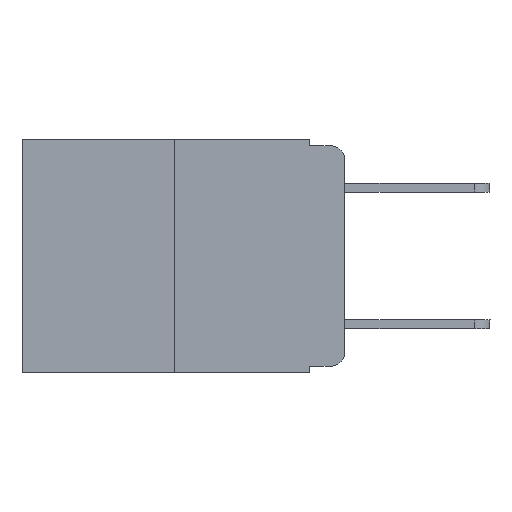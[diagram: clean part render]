
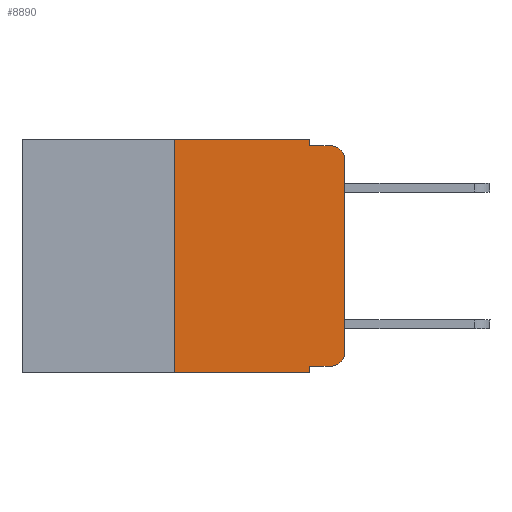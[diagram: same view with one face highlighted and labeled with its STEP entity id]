
A CAD part, left-side view. The second image highlights one B-rep face of the part: STEP entity #8890.
In plain terms, the highlighted planar face has unit normal (-1, 0, 0).
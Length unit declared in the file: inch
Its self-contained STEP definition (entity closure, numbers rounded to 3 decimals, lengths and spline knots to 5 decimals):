
#1074 = VERTEX_POINT ( 'NONE', #18819 ) ;
#1126 = VERTEX_POINT ( 'NONE', #11155 ) ;
#1210 = ORIENTED_EDGE ( 'NONE', *, *, #6990, .T. ) ;
#1225 = ORIENTED_EDGE ( 'NONE', *, *, #2847, .F. ) ;
#1250 = AXIS2_PLACEMENT_3D ( 'NONE', #14563, #1403, #7265 ) ;
#1403 = DIRECTION ( 'NONE',  ( -1., 0., 0. ) ) ;
#1538 = DIRECTION ( 'NONE',  ( 0., 0., -1. ) ) ;
#1814 = VERTEX_POINT ( 'NONE', #7582 ) ;
#2265 = DIRECTION ( 'NONE',  ( 0., 0., 1. ) ) ;
#2280 = VECTOR ( 'NONE', #1538, 39.37008 ) ;
#2627 = VERTEX_POINT ( 'NONE', #10776 ) ;
#2756 = DIRECTION ( 'NONE',  ( 0., 0., 1. ) ) ;
#2758 = CIRCLE ( 'NONE', #11976, 0.02 ) ;
#2847 = EDGE_CURVE ( 'NONE', #8914, #1814, #14785, .T. ) ;
#3296 = VECTOR ( 'NONE', #14700, 39.37008 ) ;
#3506 = EDGE_CURVE ( 'NONE', #2627, #1074, #11932, .T. ) ;
#3644 = ORIENTED_EDGE ( 'NONE', *, *, #6908, .F. ) ;
#3675 = VECTOR ( 'NONE', #2265, 39.37008 ) ;
#3676 = DIRECTION ( 'NONE',  ( 0., 0., -1. ) ) ;
#3767 = CARTESIAN_POINT ( 'NONE',  ( 0., 0.051, 0. ) ) ;
#4050 = VECTOR ( 'NONE', #14196, 39.37008 ) ;
#4240 = EDGE_CURVE ( 'NONE', #1814, #13619, #12822, .T. ) ;
#4284 = VECTOR ( 'NONE', #6606, 39.37008 ) ;
#4332 = EDGE_CURVE ( 'NONE', #8273, #1126, #2758, .T. ) ;
#4695 = ORIENTED_EDGE ( 'NONE', *, *, #4332, .T. ) ;
#5544 = CARTESIAN_POINT ( 'NONE',  ( 0., 0., 0. ) ) ;
#5712 = EDGE_CURVE ( 'NONE', #12808, #13619, #15641, .T. ) ;
#6107 = ORIENTED_EDGE ( 'NONE', *, *, #12561, .F. ) ;
#6126 = CARTESIAN_POINT ( 'NONE',  ( 0., 0., -0.03 ) ) ;
#6606 = DIRECTION ( 'NONE',  ( 0., -1., 0. ) ) ;
#6854 = LINE ( 'NONE', #11003, #3675 ) ;
#6908 = EDGE_CURVE ( 'NONE', #9646, #8914, #10864, .T. ) ;
#6912 = ORIENTED_EDGE ( 'NONE', *, *, #15913, .T. ) ;
#6990 = EDGE_CURVE ( 'NONE', #1126, #12808, #18689, .T. ) ;
#7215 = CARTESIAN_POINT ( 'NONE',  ( 0., 0.02, -0.01 ) ) ;
#7265 = DIRECTION ( 'NONE',  ( 0., 0., -1. ) ) ;
#7306 = ORIENTED_EDGE ( 'NONE', *, *, #5712, .T. ) ;
#7422 = VECTOR ( 'NONE', #2756, 39.37008 ) ;
#7582 = CARTESIAN_POINT ( 'NONE',  ( 0., 0.051, -0.01 ) ) ;
#8104 = CARTESIAN_POINT ( 'NONE',  ( 0., 0.02, -0.333 ) ) ;
#8273 = VERTEX_POINT ( 'NONE', #8104 ) ;
#8346 = DIRECTION ( 'NONE',  ( 0., -1., 0. ) ) ;
#8890 = ADVANCED_FACE ( 'NONE', ( #9974 ), #12957, .F. ) ;
#8914 = VERTEX_POINT ( 'NONE', #13253 ) ;
#9047 = CARTESIAN_POINT ( 'NONE',  ( 0., 0.473, -0.343 ) ) ;
#9646 = VERTEX_POINT ( 'NONE', #18299 ) ;
#9685 = LINE ( 'NONE', #11042, #12811 ) ;
#9974 = FACE_OUTER_BOUND ( 'NONE', #17693, .T. ) ;
#10221 = ORIENTED_EDGE ( 'NONE', *, *, #4240, .F. ) ;
#10776 = CARTESIAN_POINT ( 'NONE',  ( 0., 0.25, -0.343 ) ) ;
#10864 = LINE ( 'NONE', #14278, #4050 ) ;
#11003 = CARTESIAN_POINT ( 'NONE',  ( 0., 0.25, 0. ) ) ;
#11042 = CARTESIAN_POINT ( 'NONE',  ( 0., 0.051, -0.333 ) ) ;
#11155 = CARTESIAN_POINT ( 'NONE',  ( 0., 0., -0.313 ) ) ;
#11304 = DIRECTION ( 'NONE',  ( -1., 0., 0. ) ) ;
#11352 = ORIENTED_EDGE ( 'NONE', *, *, #3506, .T. ) ;
#11932 = LINE ( 'NONE', #9047, #3296 ) ;
#11976 = AXIS2_PLACEMENT_3D ( 'NONE', #18591, #11304, #14096 ) ;
#12561 = EDGE_CURVE ( 'NONE', #17718, #1074, #15547, .T. ) ;
#12744 = AXIS2_PLACEMENT_3D ( 'NONE', #18805, #15837, #16325 ) ;
#12808 = VERTEX_POINT ( 'NONE', #6126 ) ;
#12811 = VECTOR ( 'NONE', #8346, 39.37008 ) ;
#12822 = LINE ( 'NONE', #15429, #4284 ) ;
#12957 = PLANE ( 'NONE',  #12744 ) ;
#13253 = CARTESIAN_POINT ( 'NONE',  ( 0., 0.051, 0. ) ) ;
#13619 = VERTEX_POINT ( 'NONE', #7215 ) ;
#14096 = DIRECTION ( 'NONE',  ( 0., 0., -1. ) ) ;
#14196 = DIRECTION ( 'NONE',  ( 0., -1., 0. ) ) ;
#14258 = VECTOR ( 'NONE', #3676, 39.37008 ) ;
#14278 = CARTESIAN_POINT ( 'NONE',  ( 0., 0.473, 0. ) ) ;
#14563 = CARTESIAN_POINT ( 'NONE',  ( 0., 0.02, -0.03 ) ) ;
#14700 = DIRECTION ( 'NONE',  ( 0., -1., 0. ) ) ;
#14785 = LINE ( 'NONE', #18900, #2280 ) ;
#15429 = CARTESIAN_POINT ( 'NONE',  ( 0., 0.051, -0.01 ) ) ;
#15547 = LINE ( 'NONE', #3767, #14258 ) ;
#15641 = CIRCLE ( 'NONE', #1250, 0.02 ) ;
#15837 = DIRECTION ( 'NONE',  ( 1., 0., 0. ) ) ;
#15913 = EDGE_CURVE ( 'NONE', #17718, #8273, #9685, .T. ) ;
#16325 = DIRECTION ( 'NONE',  ( 0., 0., -1. ) ) ;
#16658 = ORIENTED_EDGE ( 'NONE', *, *, #18131, .F. ) ;
#17052 = CARTESIAN_POINT ( 'NONE',  ( 0., 0.051, -0.333 ) ) ;
#17693 = EDGE_LOOP ( 'NONE', ( #1210, #7306, #10221, #1225, #3644, #16658, #11352, #6107, #6912, #4695 ) ) ;
#17718 = VERTEX_POINT ( 'NONE', #17052 ) ;
#18131 = EDGE_CURVE ( 'NONE', #2627, #9646, #6854, .T. ) ;
#18299 = CARTESIAN_POINT ( 'NONE',  ( 0., 0.25, 0. ) ) ;
#18591 = CARTESIAN_POINT ( 'NONE',  ( 0., 0.02, -0.313 ) ) ;
#18689 = LINE ( 'NONE', #5544, #7422 ) ;
#18805 = CARTESIAN_POINT ( 'NONE',  ( 0., 0.473, 0. ) ) ;
#18819 = CARTESIAN_POINT ( 'NONE',  ( 0., 0.051, -0.343 ) ) ;
#18900 = CARTESIAN_POINT ( 'NONE',  ( 0., 0.051, 0. ) ) ;
